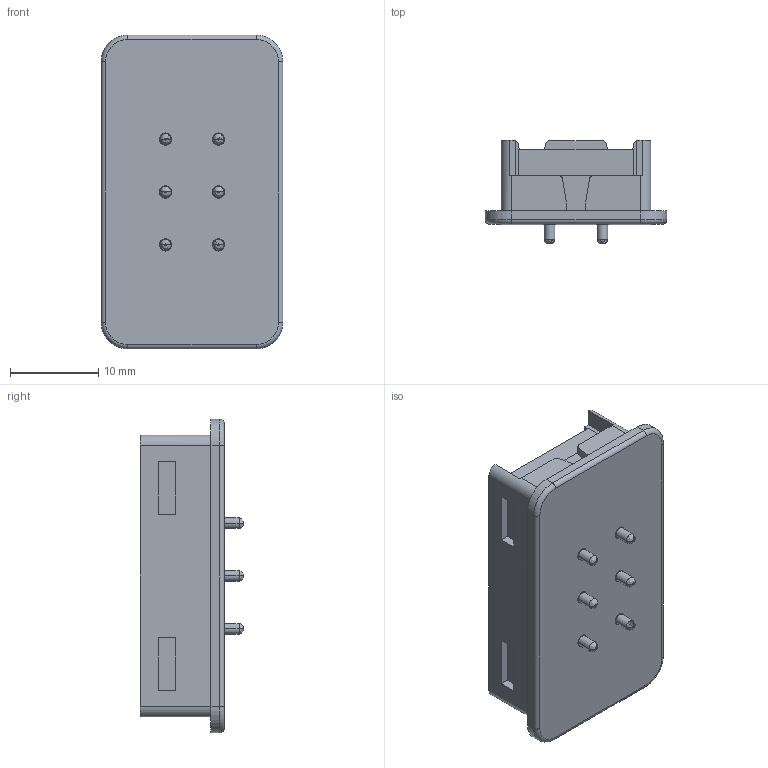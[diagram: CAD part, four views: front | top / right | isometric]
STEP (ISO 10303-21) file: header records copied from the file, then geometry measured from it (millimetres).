
FILE_DESCRIPTION (( 'STEP AP203' ), '1' );
FILE_NAME ('685-C06B1261110.STEP', '2023-02-13T13:18:08', ( 'Magnum' ), ( '' ), 'SwSTEP 2.0', 'SolidWorks 2020', '' );
FILE_SCHEMA (( 'CONFIG_CONTROL_DESIGN' ));
Length unit declared in the file: millimetre
Products named in the file (1): 685-C06B1261110
Bounding box: 20.6 x 11.7 x 35.6 mm (x, y, z)
Volume: 3744.1 mm3; surface area: 3558.4 mm2
Topology: 7 solids, 12 shells, 347 faces, 845 edges, 540 vertices
Faces by surface type: plane 190, cylinder 115, cone 22, bspline 16, torus 4
Entity records: 10694 total; most frequent: CARTESIAN_POINT 2321, DIRECTION 1793, ORIENTED_EDGE 1666, EDGE_CURVE 833, AXIS2_PLACEMENT_3D 652, VERTEX_POINT 540, VECTOR 489, LINE 489
